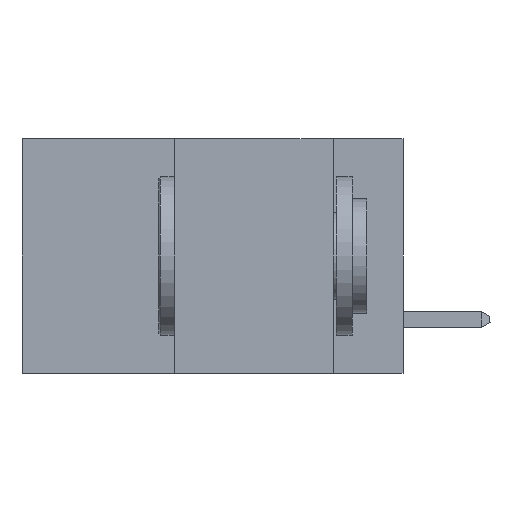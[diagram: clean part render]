
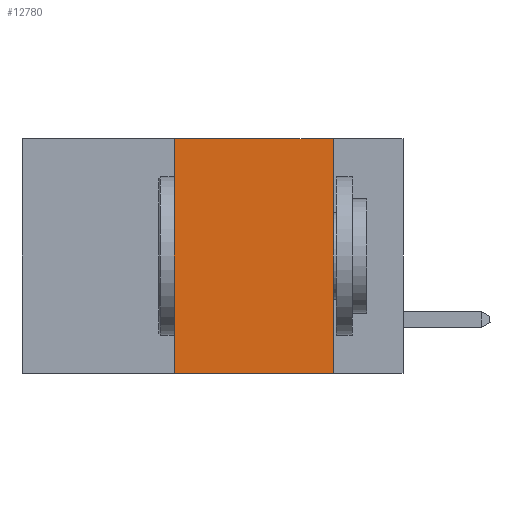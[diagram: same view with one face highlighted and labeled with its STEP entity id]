
A CAD part, left-side view. The second image highlights one B-rep face of the part: STEP entity #12780.
In plain terms, the highlighted planar face has unit normal (-1, 0, 0).
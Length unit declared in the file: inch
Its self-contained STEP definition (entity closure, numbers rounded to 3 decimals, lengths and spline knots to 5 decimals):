
#2097 = CARTESIAN_POINT ( 'NONE',  ( 0., 0.6, 0. ) ) ;
#4997 = VERTEX_POINT ( 'NONE', #34040 ) ;
#6155 = VERTEX_POINT ( 'NONE', #14343 ) ;
#6648 = VECTOR ( 'NONE', #7937, 39.37008 ) ;
#7937 = DIRECTION ( 'NONE',  ( 0., -1., 0. ) ) ;
#8062 = DIRECTION ( 'NONE',  ( 0., 0., -1. ) ) ;
#9147 = VECTOR ( 'NONE', #20734, 39.37008 ) ;
#12780 = ADVANCED_FACE ( 'NONE', ( #25127 ), #16516, .F. ) ;
#14343 = CARTESIAN_POINT ( 'NONE',  ( 0., 0.36, 0. ) ) ;
#14562 = CARTESIAN_POINT ( 'NONE',  ( 0., 0.6, -0.37 ) ) ;
#15840 = EDGE_CURVE ( 'NONE', #21535, #4997, #22289, .T. ) ;
#16092 = CARTESIAN_POINT ( 'NONE',  ( 0., 0.36, -0.37 ) ) ;
#16516 = PLANE ( 'NONE',  #22794 ) ;
#18984 = LINE ( 'NONE', #45221, #9147 ) ;
#20734 = DIRECTION ( 'NONE',  ( 0., 0., 1. ) ) ;
#21535 = VERTEX_POINT ( 'NONE', #35451 ) ;
#21667 = ORIENTED_EDGE ( 'NONE', *, *, #24921, .T. ) ;
#22104 = EDGE_CURVE ( 'NONE', #22747, #6155, #18984, .T. ) ;
#22289 = LINE ( 'NONE', #36521, #28062 ) ;
#22747 = VERTEX_POINT ( 'NONE', #16092 ) ;
#22794 = AXIS2_PLACEMENT_3D ( 'NONE', #2097, #42307, #31698 ) ;
#24921 = EDGE_CURVE ( 'NONE', #22747, #4997, #32549, .T. ) ;
#25127 = FACE_OUTER_BOUND ( 'NONE', #42324, .T. ) ;
#28062 = VECTOR ( 'NONE', #8062, 39.37008 ) ;
#28452 = ORIENTED_EDGE ( 'NONE', *, *, #22104, .F. ) ;
#31698 = DIRECTION ( 'NONE',  ( 0., 0., -1. ) ) ;
#32549 = LINE ( 'NONE', #14562, #44637 ) ;
#33131 = ORIENTED_EDGE ( 'NONE', *, *, #15840, .F. ) ;
#34040 = CARTESIAN_POINT ( 'NONE',  ( 0., 0.11, -0.37 ) ) ;
#35451 = CARTESIAN_POINT ( 'NONE',  ( 0., 0.11, 0. ) ) ;
#35528 = EDGE_CURVE ( 'NONE', #6155, #21535, #41264, .T. ) ;
#35865 = DIRECTION ( 'NONE',  ( 0., -1., 0. ) ) ;
#36521 = CARTESIAN_POINT ( 'NONE',  ( 0., 0.11, 0. ) ) ;
#37978 = ORIENTED_EDGE ( 'NONE', *, *, #35528, .F. ) ;
#41264 = LINE ( 'NONE', #45073, #6648 ) ;
#42307 = DIRECTION ( 'NONE',  ( 1., 0., 0. ) ) ;
#42324 = EDGE_LOOP ( 'NONE', ( #33131, #37978, #28452, #21667 ) ) ;
#44637 = VECTOR ( 'NONE', #35865, 39.37008 ) ;
#45073 = CARTESIAN_POINT ( 'NONE',  ( 0., 0.6, 0. ) ) ;
#45221 = CARTESIAN_POINT ( 'NONE',  ( 0., 0.36, 0. ) ) ;
